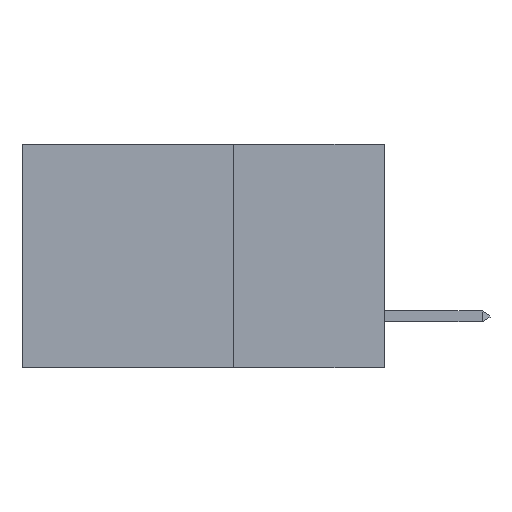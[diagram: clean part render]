
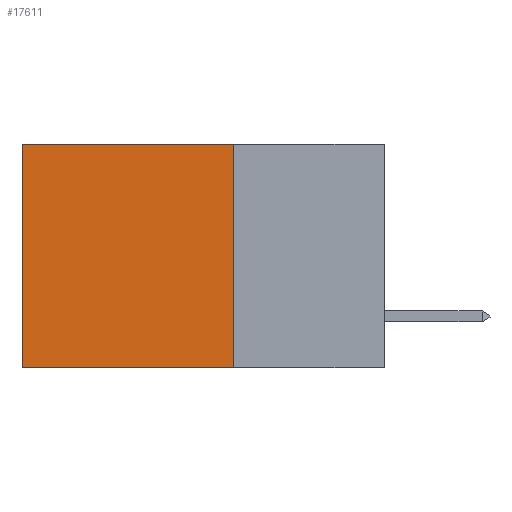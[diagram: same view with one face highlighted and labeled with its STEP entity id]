
A CAD part, left-side view. The second image highlights one B-rep face of the part: STEP entity #17611.
In plain terms, the highlighted planar face has unit normal (-1, 0, 0).
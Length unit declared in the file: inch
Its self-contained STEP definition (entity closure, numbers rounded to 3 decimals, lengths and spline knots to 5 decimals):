
#1071 = EDGE_CURVE ( 'NONE', #8227, #10710, #18184, .T. ) ;
#1091 = CARTESIAN_POINT ( 'NONE',  ( 0.2875, 0.25, 0. ) ) ;
#2144 = ORIENTED_EDGE ( 'NONE', *, *, #1071, .T. ) ;
#2977 = DIRECTION ( 'NONE',  ( 0., 0., -1. ) ) ;
#3110 = CARTESIAN_POINT ( 'NONE',  ( 0.2875, 0.25, -0.37 ) ) ;
#3461 = VERTEX_POINT ( 'NONE', #10325 ) ;
#3834 = ORIENTED_EDGE ( 'NONE', *, *, #12022, .F. ) ;
#3904 = AXIS2_PLACEMENT_3D ( 'NONE', #1091, #14214, #2977 ) ;
#4406 = CARTESIAN_POINT ( 'NONE',  ( 0.2875, 0.25, 0. ) ) ;
#4607 = LINE ( 'NONE', #7027, #18957 ) ;
#4985 = VECTOR ( 'NONE', #23554, 39.37008 ) ;
#6229 = ORIENTED_EDGE ( 'NONE', *, *, #22958, .F. ) ;
#7027 = CARTESIAN_POINT ( 'NONE',  ( 0.2875, 0.25, 0. ) ) ;
#8227 = VERTEX_POINT ( 'NONE', #4406 ) ;
#8254 = VECTOR ( 'NONE', #19760, 39.37008 ) ;
#9465 = LINE ( 'NONE', #18758, #23738 ) ;
#10325 = CARTESIAN_POINT ( 'NONE',  ( 0.2875, 0.6, -0.37 ) ) ;
#10474 = PLANE ( 'NONE',  #3904 ) ;
#10710 = VERTEX_POINT ( 'NONE', #16181 ) ;
#11025 = CARTESIAN_POINT ( 'NONE',  ( 0.2875, 0.25, -0.37 ) ) ;
#11281 = DIRECTION ( 'NONE',  ( 0., 0., -1. ) ) ;
#11440 = VERTEX_POINT ( 'NONE', #11025 ) ;
#12022 = EDGE_CURVE ( 'NONE', #8227, #11440, #4607, .T. ) ;
#12710 = FACE_OUTER_BOUND ( 'NONE', #13440, .T. ) ;
#13440 = EDGE_LOOP ( 'NONE', ( #23421, #6229, #3834, #2144 ) ) ;
#14214 = DIRECTION ( 'NONE',  ( 1., 0., 0. ) ) ;
#14383 = LINE ( 'NONE', #3110, #4985 ) ;
#16181 = CARTESIAN_POINT ( 'NONE',  ( 0.2875, 0.6, 0. ) ) ;
#16446 = DIRECTION ( 'NONE',  ( 0., 0., -1. ) ) ;
#17611 = ADVANCED_FACE ( 'NONE', ( #12710 ), #10474, .F. ) ;
#18184 = LINE ( 'NONE', #21637, #8254 ) ;
#18758 = CARTESIAN_POINT ( 'NONE',  ( 0.2875, 0.6, 0. ) ) ;
#18957 = VECTOR ( 'NONE', #16446, 39.37008 ) ;
#19760 = DIRECTION ( 'NONE',  ( 0., 1., 0. ) ) ;
#21637 = CARTESIAN_POINT ( 'NONE',  ( 0.2875, 0.25, 0. ) ) ;
#22571 = EDGE_CURVE ( 'NONE', #10710, #3461, #9465, .T. ) ;
#22958 = EDGE_CURVE ( 'NONE', #11440, #3461, #14383, .T. ) ;
#23421 = ORIENTED_EDGE ( 'NONE', *, *, #22571, .T. ) ;
#23554 = DIRECTION ( 'NONE',  ( 0., 1., 0. ) ) ;
#23738 = VECTOR ( 'NONE', #11281, 39.37008 ) ;
